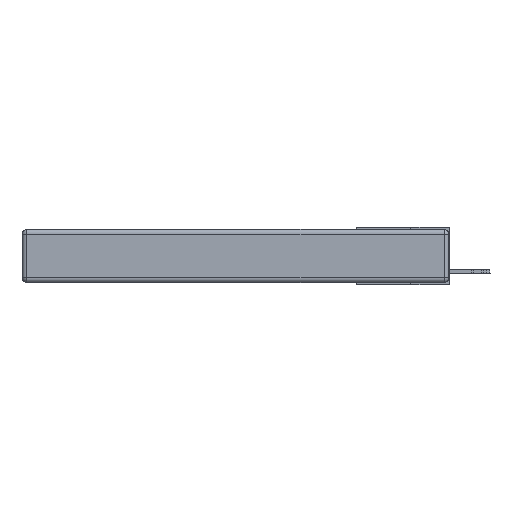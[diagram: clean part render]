
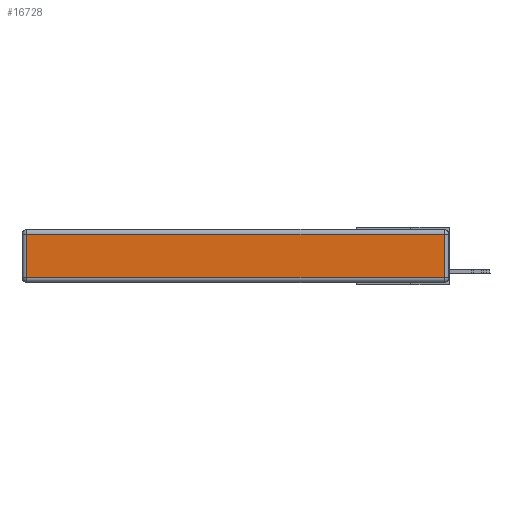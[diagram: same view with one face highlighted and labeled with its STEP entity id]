
A CAD part, left-side view. The second image highlights one B-rep face of the part: STEP entity #16728.
In plain terms, the highlighted planar face has unit normal (-1, 0, 0).
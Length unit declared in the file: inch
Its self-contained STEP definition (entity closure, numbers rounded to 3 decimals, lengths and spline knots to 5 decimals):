
#693 = LINE ( 'NONE', #7104, #26759 ) ;
#1226 = ORIENTED_EDGE ( 'NONE', *, *, #32670, .T. ) ;
#1452 = VECTOR ( 'NONE', #25471, 39.37008 ) ;
#1920 = EDGE_LOOP ( 'NONE', ( #27307, #12866, #1226, #32325 ) ) ;
#3125 = CARTESIAN_POINT ( 'NONE',  ( 0., 2.75, -0.03 ) ) ;
#3232 = CARTESIAN_POINT ( 'NONE',  ( 0., 0.03, -0.03 ) ) ;
#4470 = VERTEX_POINT ( 'NONE', #13143 ) ;
#7104 = CARTESIAN_POINT ( 'NONE',  ( 0., 0., -0.313 ) ) ;
#7205 = DIRECTION ( 'NONE',  ( 0., 0., 1. ) ) ;
#7744 = DIRECTION ( 'NONE',  ( 0., 1., 0. ) ) ;
#7989 = CARTESIAN_POINT ( 'NONE',  ( 0., 2.72, -0.343 ) ) ;
#9925 = EDGE_CURVE ( 'NONE', #15163, #4470, #10520, .T. ) ;
#10520 = LINE ( 'NONE', #7989, #1452 ) ;
#11528 = LINE ( 'NONE', #15045, #28552 ) ;
#12100 = EDGE_CURVE ( 'NONE', #14222, #19536, #11528, .T. ) ;
#12790 = CARTESIAN_POINT ( 'NONE',  ( 0., 2.72, -0.03 ) ) ;
#12866 = ORIENTED_EDGE ( 'NONE', *, *, #12100, .T. ) ;
#13143 = CARTESIAN_POINT ( 'NONE',  ( 0., 2.72, -0.313 ) ) ;
#14222 = VERTEX_POINT ( 'NONE', #22137 ) ;
#15045 = CARTESIAN_POINT ( 'NONE',  ( 0., 0.03, -0.343 ) ) ;
#15163 = VERTEX_POINT ( 'NONE', #12790 ) ;
#16728 = ADVANCED_FACE ( 'NONE', ( #25680 ), #32025, .T. ) ;
#16916 = CARTESIAN_POINT ( 'NONE',  ( 0., 0., -0.343 ) ) ;
#18160 = VECTOR ( 'NONE', #7744, 39.37008 ) ;
#18288 = EDGE_CURVE ( 'NONE', #4470, #14222, #693, .T. ) ;
#19499 = DIRECTION ( 'NONE',  ( 0., -1., 0. ) ) ;
#19536 = VERTEX_POINT ( 'NONE', #3232 ) ;
#21114 = AXIS2_PLACEMENT_3D ( 'NONE', #16916, #24533, #29416 ) ;
#22137 = CARTESIAN_POINT ( 'NONE',  ( 0., 0.03, -0.313 ) ) ;
#24533 = DIRECTION ( 'NONE',  ( -1., 0., 0. ) ) ;
#25471 = DIRECTION ( 'NONE',  ( 0., 0., -1. ) ) ;
#25680 = FACE_OUTER_BOUND ( 'NONE', #1920, .T. ) ;
#26759 = VECTOR ( 'NONE', #19499, 39.37008 ) ;
#27307 = ORIENTED_EDGE ( 'NONE', *, *, #18288, .T. ) ;
#28552 = VECTOR ( 'NONE', #7205, 39.37008 ) ;
#29416 = DIRECTION ( 'NONE',  ( 0., 0., 1. ) ) ;
#31576 = LINE ( 'NONE', #3125, #18160 ) ;
#32025 = PLANE ( 'NONE',  #21114 ) ;
#32325 = ORIENTED_EDGE ( 'NONE', *, *, #9925, .T. ) ;
#32670 = EDGE_CURVE ( 'NONE', #19536, #15163, #31576, .T. ) ;
